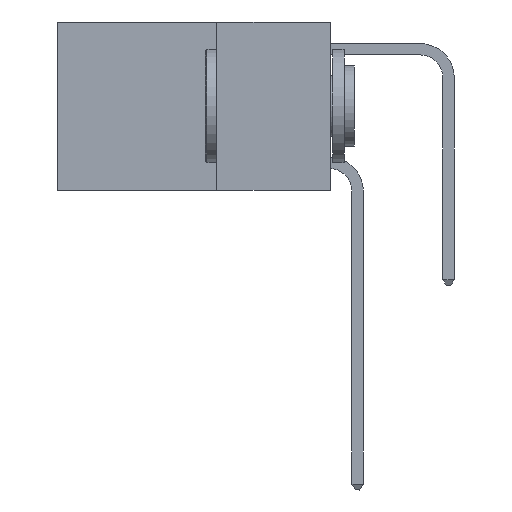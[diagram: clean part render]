
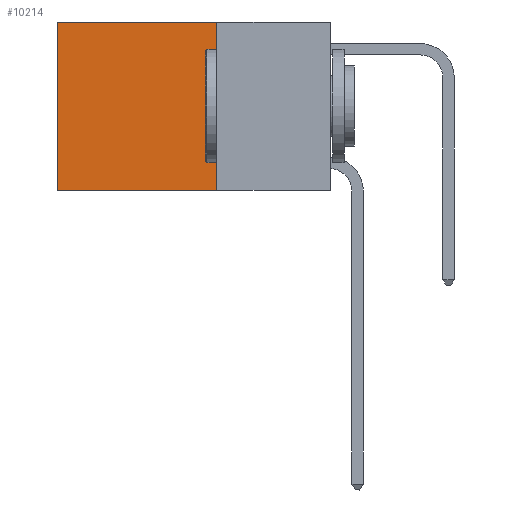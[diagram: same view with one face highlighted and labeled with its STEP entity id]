
A CAD part, left-side view. The second image highlights one B-rep face of the part: STEP entity #10214.
In plain terms, the highlighted planar face has unit normal (-1, 0, 0).
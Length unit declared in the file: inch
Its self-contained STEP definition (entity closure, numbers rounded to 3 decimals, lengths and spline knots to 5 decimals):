
#464 = VERTEX_POINT ( 'NONE', #16898 ) ;
#2575 = LINE ( 'NONE', #5838, #13090 ) ;
#2717 = DIRECTION ( 'NONE',  ( 0., 0., -1. ) ) ;
#2770 = LINE ( 'NONE', #17700, #10429 ) ;
#2781 = EDGE_LOOP ( 'NONE', ( #10955, #12244, #12423, #8016 ) ) ;
#3413 = VERTEX_POINT ( 'NONE', #12184 ) ;
#5605 = CARTESIAN_POINT ( 'NONE',  ( 0.2625, 0.25, 0. ) ) ;
#5838 = CARTESIAN_POINT ( 'NONE',  ( 0.2625, 0.25, -0.37 ) ) ;
#6524 = AXIS2_PLACEMENT_3D ( 'NONE', #17241, #7255, #17297 ) ;
#7255 = DIRECTION ( 'NONE',  ( 1., 0., 0. ) ) ;
#7674 = LINE ( 'NONE', #5605, #14803 ) ;
#7767 = LINE ( 'NONE', #8540, #11118 ) ;
#8016 = ORIENTED_EDGE ( 'NONE', *, *, #11982, .T. ) ;
#8539 = EDGE_CURVE ( 'NONE', #3413, #464, #7674, .T. ) ;
#8540 = CARTESIAN_POINT ( 'NONE',  ( 0.2625, 0.25, 0. ) ) ;
#9097 = CARTESIAN_POINT ( 'NONE',  ( 0.2625, 0.6, -0.37 ) ) ;
#9876 = FACE_OUTER_BOUND ( 'NONE', #2781, .T. ) ;
#10214 = ADVANCED_FACE ( 'NONE', ( #9876 ), #15839, .F. ) ;
#10429 = VECTOR ( 'NONE', #10574, 39.37008 ) ;
#10574 = DIRECTION ( 'NONE',  ( 0., 0., -1. ) ) ;
#10955 = ORIENTED_EDGE ( 'NONE', *, *, #13487, .T. ) ;
#11118 = VECTOR ( 'NONE', #15654, 39.37008 ) ;
#11543 = VERTEX_POINT ( 'NONE', #16108 ) ;
#11982 = EDGE_CURVE ( 'NONE', #3413, #11543, #7767, .T. ) ;
#12184 = CARTESIAN_POINT ( 'NONE',  ( 0.2625, 0.25, 0. ) ) ;
#12244 = ORIENTED_EDGE ( 'NONE', *, *, #16622, .F. ) ;
#12423 = ORIENTED_EDGE ( 'NONE', *, *, #8539, .F. ) ;
#13090 = VECTOR ( 'NONE', #15880, 39.37008 ) ;
#13487 = EDGE_CURVE ( 'NONE', #11543, #18146, #2770, .T. ) ;
#14803 = VECTOR ( 'NONE', #2717, 39.37008 ) ;
#15654 = DIRECTION ( 'NONE',  ( 0., 1., 0. ) ) ;
#15839 = PLANE ( 'NONE',  #6524 ) ;
#15880 = DIRECTION ( 'NONE',  ( 0., 1., 0. ) ) ;
#16108 = CARTESIAN_POINT ( 'NONE',  ( 0.2625, 0.6, 0. ) ) ;
#16622 = EDGE_CURVE ( 'NONE', #464, #18146, #2575, .T. ) ;
#16898 = CARTESIAN_POINT ( 'NONE',  ( 0.2625, 0.25, -0.37 ) ) ;
#17241 = CARTESIAN_POINT ( 'NONE',  ( 0.2625, 0.25, 0. ) ) ;
#17297 = DIRECTION ( 'NONE',  ( 0., 0., -1. ) ) ;
#17700 = CARTESIAN_POINT ( 'NONE',  ( 0.2625, 0.6, 0. ) ) ;
#18146 = VERTEX_POINT ( 'NONE', #9097 ) ;
